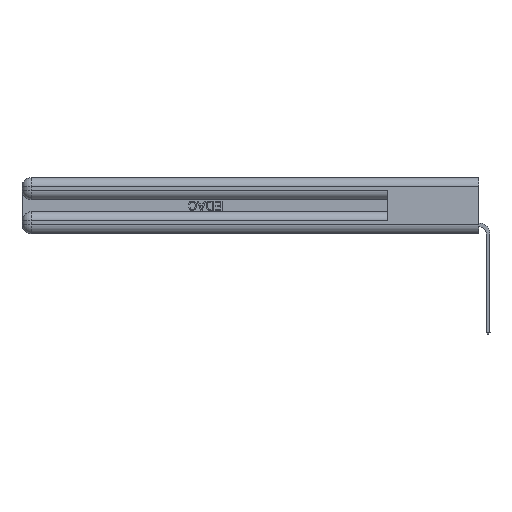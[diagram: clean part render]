
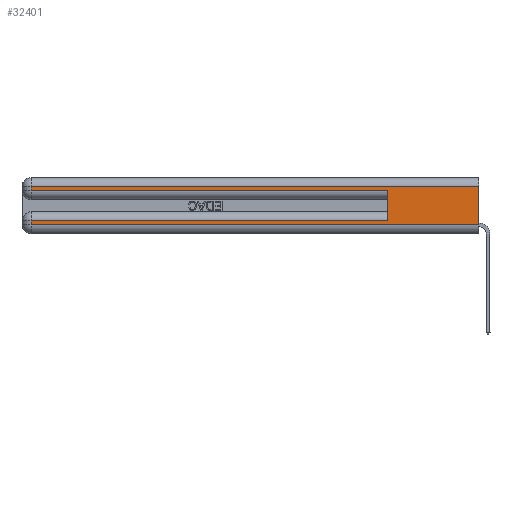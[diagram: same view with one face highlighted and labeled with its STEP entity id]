
A CAD part, left-side view. The second image highlights one B-rep face of the part: STEP entity #32401.
In plain terms, the highlighted planar face has unit normal (-1, 0, 0).
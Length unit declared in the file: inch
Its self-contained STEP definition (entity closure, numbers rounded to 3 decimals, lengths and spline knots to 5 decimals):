
#1185 = CARTESIAN_POINT ( 'NONE',  ( 0., 0., 0.06 ) ) ;
#1320 = AXIS2_PLACEMENT_3D ( 'NONE', #22968, #18062, #2561 ) ;
#1751 = DIRECTION ( 'NONE',  ( 0., -1., 0. ) ) ;
#2527 = ORIENTED_EDGE ( 'NONE', *, *, #24724, .T. ) ;
#2561 = DIRECTION ( 'NONE',  ( 0., 0., -1. ) ) ;
#2892 = VERTEX_POINT ( 'NONE', #8747 ) ;
#3399 = EDGE_CURVE ( 'NONE', #28226, #16261, #25229, .T. ) ;
#4400 = CARTESIAN_POINT ( 'NONE',  ( 0., 0., 0.37 ) ) ;
#4465 = VERTEX_POINT ( 'NONE', #23796 ) ;
#5413 = CARTESIAN_POINT ( 'NONE',  ( 0., 0.6, 0.285 ) ) ;
#5653 = VERTEX_POINT ( 'NONE', #5413 ) ;
#7123 = CARTESIAN_POINT ( 'NONE',  ( 0., 2.94, 0.285 ) ) ;
#7206 = LINE ( 'NONE', #8969, #13288 ) ;
#7437 = LINE ( 'NONE', #14987, #21133 ) ;
#7765 = ORIENTED_EDGE ( 'NONE', *, *, #29889, .T. ) ;
#7948 = CARTESIAN_POINT ( 'NONE',  ( 0., 2.94, 0.085 ) ) ;
#8646 = ORIENTED_EDGE ( 'NONE', *, *, #19644, .T. ) ;
#8747 = CARTESIAN_POINT ( 'NONE',  ( 0., 0.6, 0.085 ) ) ;
#8955 = VECTOR ( 'NONE', #13798, 39.37008 ) ;
#8969 = CARTESIAN_POINT ( 'NONE',  ( 0., 0., 0.085 ) ) ;
#9193 = ORIENTED_EDGE ( 'NONE', *, *, #14481, .T. ) ;
#9858 = LINE ( 'NONE', #26793, #25086 ) ;
#10998 = EDGE_CURVE ( 'NONE', #4465, #16261, #9858, .T. ) ;
#11465 = DIRECTION ( 'NONE',  ( 0., -1., 0. ) ) ;
#13288 = VECTOR ( 'NONE', #16795, 39.37008 ) ;
#13627 = CARTESIAN_POINT ( 'NONE',  ( 0., 0., 0.31 ) ) ;
#13673 = ORIENTED_EDGE ( 'NONE', *, *, #10998, .T. ) ;
#13798 = DIRECTION ( 'NONE',  ( 0., 0., -1. ) ) ;
#14481 = EDGE_CURVE ( 'NONE', #16593, #4465, #7437, .T. ) ;
#14880 = VECTOR ( 'NONE', #21360, 39.37008 ) ;
#14937 = ORIENTED_EDGE ( 'NONE', *, *, #33290, .T. ) ;
#14987 = CARTESIAN_POINT ( 'NONE',  ( 0., 2.94, 0.37 ) ) ;
#15308 = ORIENTED_EDGE ( 'NONE', *, *, #21334, .F. ) ;
#15490 = PLANE ( 'NONE',  #1320 ) ;
#15871 = LINE ( 'NONE', #29103, #8955 ) ;
#16261 = VERTEX_POINT ( 'NONE', #1185 ) ;
#16593 = VERTEX_POINT ( 'NONE', #7948 ) ;
#16795 = DIRECTION ( 'NONE',  ( 0., 1., 0. ) ) ;
#18062 = DIRECTION ( 'NONE',  ( 1., 0., 0. ) ) ;
#19630 = EDGE_LOOP ( 'NONE', ( #21291, #14937, #7765, #2527, #15308, #8646, #9193, #13673 ) ) ;
#19644 = EDGE_CURVE ( 'NONE', #2892, #16593, #7206, .T. ) ;
#20476 = FACE_OUTER_BOUND ( 'NONE', #19630, .T. ) ;
#21133 = VECTOR ( 'NONE', #32841, 39.37008 ) ;
#21291 = ORIENTED_EDGE ( 'NONE', *, *, #3399, .F. ) ;
#21334 = EDGE_CURVE ( 'NONE', #2892, #5653, #29561, .T. ) ;
#21360 = DIRECTION ( 'NONE',  ( 0., 1., 0. ) ) ;
#21741 = CARTESIAN_POINT ( 'NONE',  ( 0., 2.94, 0.31 ) ) ;
#21965 = CARTESIAN_POINT ( 'NONE',  ( 0., 0., 0.31 ) ) ;
#22968 = CARTESIAN_POINT ( 'NONE',  ( 0., 0., 0.37 ) ) ;
#23628 = VECTOR ( 'NONE', #24953, 39.37008 ) ;
#23796 = CARTESIAN_POINT ( 'NONE',  ( 0., 2.94, 0.06 ) ) ;
#23916 = CARTESIAN_POINT ( 'NONE',  ( 0., 0.6, 0.145 ) ) ;
#24021 = DIRECTION ( 'NONE',  ( 0., 0., 1. ) ) ;
#24724 = EDGE_CURVE ( 'NONE', #31791, #5653, #27321, .T. ) ;
#24953 = DIRECTION ( 'NONE',  ( 0., 0., -1. ) ) ;
#25086 = VECTOR ( 'NONE', #11465, 39.37008 ) ;
#25229 = LINE ( 'NONE', #4400, #23628 ) ;
#26495 = VECTOR ( 'NONE', #1751, 39.37008 ) ;
#26793 = CARTESIAN_POINT ( 'NONE',  ( 0., 0., 0.06 ) ) ;
#27321 = LINE ( 'NONE', #32542, #26495 ) ;
#27952 = VECTOR ( 'NONE', #24021, 39.37008 ) ;
#28226 = VERTEX_POINT ( 'NONE', #21965 ) ;
#28435 = LINE ( 'NONE', #13627, #14880 ) ;
#29103 = CARTESIAN_POINT ( 'NONE',  ( 0., 2.94, 0.37 ) ) ;
#29561 = LINE ( 'NONE', #23916, #27952 ) ;
#29889 = EDGE_CURVE ( 'NONE', #29970, #31791, #15871, .T. ) ;
#29970 = VERTEX_POINT ( 'NONE', #21741 ) ;
#31791 = VERTEX_POINT ( 'NONE', #7123 ) ;
#32401 = ADVANCED_FACE ( 'NONE', ( #20476 ), #15490, .F. ) ;
#32542 = CARTESIAN_POINT ( 'NONE',  ( 0., 0., 0.285 ) ) ;
#32841 = DIRECTION ( 'NONE',  ( 0., 0., -1. ) ) ;
#33290 = EDGE_CURVE ( 'NONE', #28226, #29970, #28435, .T. ) ;
